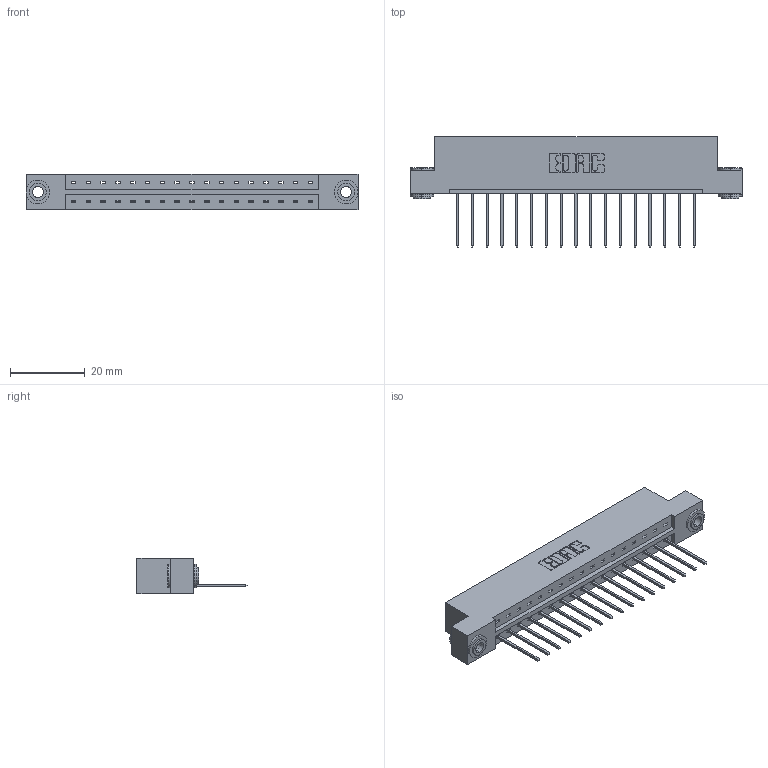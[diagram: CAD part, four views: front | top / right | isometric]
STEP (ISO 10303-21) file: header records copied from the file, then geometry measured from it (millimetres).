
FILE_DESCRIPTION (( 'STEP AP203' ), '1' );
FILE_NAME ('333-017-540-103.STEP', '2019-08-09T12:00:55', ( '' ), ( '' ), 'SwSTEP 2.0', 'SolidWorks 2016', '' );
FILE_SCHEMA (( 'CONFIG_CONTROL_DESIGN' ));
Length unit declared in the file: inch
Products named in the file (4): 345-250-002_345-250-002-102; 333 Part_Flush - .156 Dia - TH; 333-017-540-103; 345-292-001_345-293-140
Assembly tree (20 placements, depth 2):
  333-017-540-103
    333 Part_Flush - .156 Dia - TH
    345-292-001_345-293-140  x17
    345-250-002_345-250-002-102  x2
Bounding box: 88.9 x 29.47 x 9.4 mm (x, y, z)
Volume: 8773.3 mm3; surface area: 9728.3 mm2
Topology: 20 solids, 20 shells, 1138 faces, 3379 edges, 2226 vertices
Faces by surface type: plane 794, cylinder 336, cone 8
Entity records: 14294 total; most frequent: CARTESIAN_POINT 2448, ORIENTED_EDGE 2394, DIRECTION 2149, EDGE_CURVE 1197, LINE 1045, VECTOR 1045, VERTEX_POINT 794, AXIS2_PLACEMENT_3D 552
